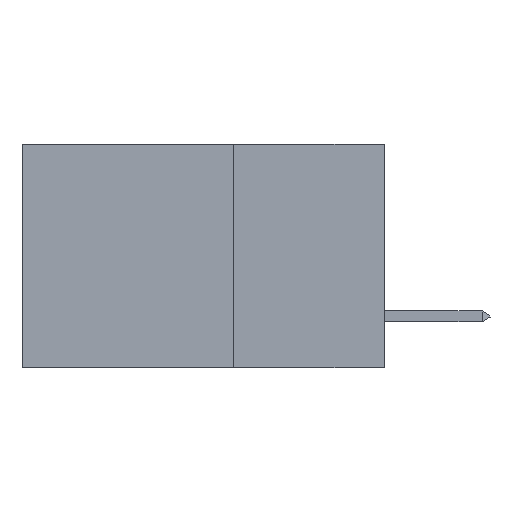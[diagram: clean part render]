
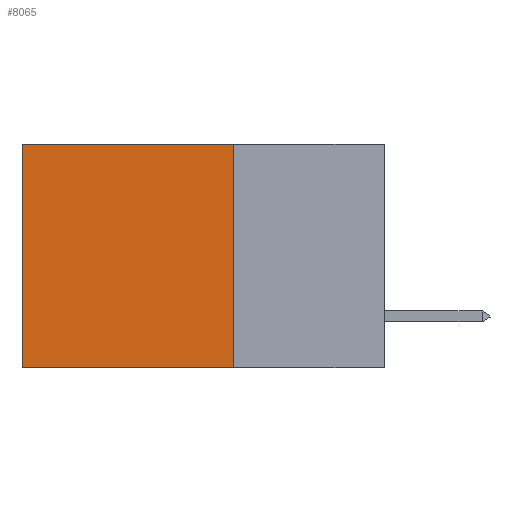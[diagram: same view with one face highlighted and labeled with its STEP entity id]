
A CAD part, left-side view. The second image highlights one B-rep face of the part: STEP entity #8065.
In plain terms, the highlighted planar face has unit normal (-1, 0, 0).
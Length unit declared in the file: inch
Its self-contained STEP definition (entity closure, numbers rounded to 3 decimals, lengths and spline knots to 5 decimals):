
#597 = CARTESIAN_POINT ( 'NONE',  ( 0.2875, 0.25, 0. ) ) ;
#1141 = VERTEX_POINT ( 'NONE', #597 ) ;
#1185 = LINE ( 'NONE', #7125, #2026 ) ;
#1737 = ORIENTED_EDGE ( 'NONE', *, *, #2357, .F. ) ;
#2026 = VECTOR ( 'NONE', #8348, 39.37008 ) ;
#2357 = EDGE_CURVE ( 'NONE', #14583, #33768, #28648, .T. ) ;
#2685 = DIRECTION ( 'NONE',  ( 0., 1., 0. ) ) ;
#4022 = DIRECTION ( 'NONE',  ( 0., 1., 0. ) ) ;
#4376 = VECTOR ( 'NONE', #4022, 39.37008 ) ;
#5552 = DIRECTION ( 'NONE',  ( 1., 0., 0. ) ) ;
#7125 = CARTESIAN_POINT ( 'NONE',  ( 0.2875, 0.25, 0. ) ) ;
#7431 = EDGE_CURVE ( 'NONE', #15432, #33768, #33912, .T. ) ;
#8065 = ADVANCED_FACE ( 'NONE', ( #23335 ), #21328, .F. ) ;
#8348 = DIRECTION ( 'NONE',  ( 0., 0., -1. ) ) ;
#8415 = EDGE_CURVE ( 'NONE', #1141, #14583, #1185, .T. ) ;
#9162 = CARTESIAN_POINT ( 'NONE',  ( 0.2875, 0.25, 0. ) ) ;
#10794 = VECTOR ( 'NONE', #24523, 39.37008 ) ;
#12567 = VECTOR ( 'NONE', #2685, 39.37008 ) ;
#13127 = CARTESIAN_POINT ( 'NONE',  ( 0.2875, 0.25, -0.37 ) ) ;
#13188 = ORIENTED_EDGE ( 'NONE', *, *, #8415, .F. ) ;
#13411 = CARTESIAN_POINT ( 'NONE',  ( 0.2875, 0.25, -0.37 ) ) ;
#13738 = CARTESIAN_POINT ( 'NONE',  ( 0.2875, 0.25, 0. ) ) ;
#14486 = ORIENTED_EDGE ( 'NONE', *, *, #21591, .T. ) ;
#14583 = VERTEX_POINT ( 'NONE', #13127 ) ;
#15432 = VERTEX_POINT ( 'NONE', #31929 ) ;
#16305 = CARTESIAN_POINT ( 'NONE',  ( 0.2875, 0.6, 0. ) ) ;
#18733 = AXIS2_PLACEMENT_3D ( 'NONE', #13738, #5552, #21522 ) ;
#21207 = CARTESIAN_POINT ( 'NONE',  ( 0.2875, 0.6, -0.37 ) ) ;
#21328 = PLANE ( 'NONE',  #18733 ) ;
#21522 = DIRECTION ( 'NONE',  ( 0., 0., -1. ) ) ;
#21591 = EDGE_CURVE ( 'NONE', #1141, #15432, #29082, .T. ) ;
#22486 = ORIENTED_EDGE ( 'NONE', *, *, #7431, .T. ) ;
#23335 = FACE_OUTER_BOUND ( 'NONE', #30045, .T. ) ;
#24523 = DIRECTION ( 'NONE',  ( 0., 0., -1. ) ) ;
#28648 = LINE ( 'NONE', #13411, #12567 ) ;
#29082 = LINE ( 'NONE', #9162, #4376 ) ;
#30045 = EDGE_LOOP ( 'NONE', ( #22486, #1737, #13188, #14486 ) ) ;
#31929 = CARTESIAN_POINT ( 'NONE',  ( 0.2875, 0.6, 0. ) ) ;
#33768 = VERTEX_POINT ( 'NONE', #21207 ) ;
#33912 = LINE ( 'NONE', #16305, #10794 ) ;
